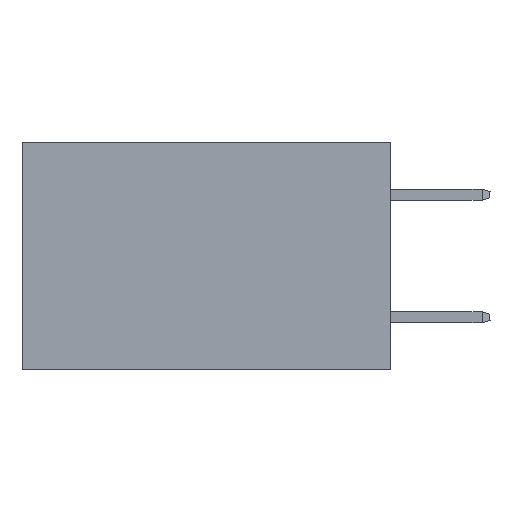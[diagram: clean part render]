
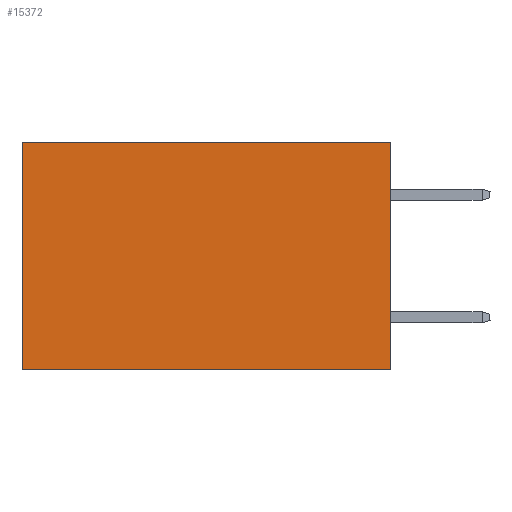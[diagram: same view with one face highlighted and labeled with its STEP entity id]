
A CAD part, left-side view. The second image highlights one B-rep face of the part: STEP entity #15372.
In plain terms, the highlighted planar face has unit normal (-1, 0, 0).
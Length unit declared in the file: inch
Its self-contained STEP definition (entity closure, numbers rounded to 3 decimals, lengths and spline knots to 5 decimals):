
#166 = CARTESIAN_POINT ( 'NONE',  ( 0.2875, 0., 0. ) ) ;
#623 = LINE ( 'NONE', #166, #16661 ) ;
#1208 = DIRECTION ( 'NONE',  ( 0., 0., -1. ) ) ;
#1688 = PLANE ( 'NONE',  #29079 ) ;
#3999 = CARTESIAN_POINT ( 'NONE',  ( 0.2875, 0., 0. ) ) ;
#4594 = EDGE_CURVE ( 'NONE', #4764, #20289, #623, .T. ) ;
#4764 = VERTEX_POINT ( 'NONE', #3999 ) ;
#5933 = ORIENTED_EDGE ( 'NONE', *, *, #18260, .F. ) ;
#6297 = CARTESIAN_POINT ( 'NONE',  ( 0.2875, 0., 0. ) ) ;
#6328 = DIRECTION ( 'NONE',  ( 0., 1., 0. ) ) ;
#7002 = CARTESIAN_POINT ( 'NONE',  ( 0.2875, 0., 0. ) ) ;
#7034 = CARTESIAN_POINT ( 'NONE',  ( 0.2875, 0., -0.37 ) ) ;
#7467 = ORIENTED_EDGE ( 'NONE', *, *, #11620, .T. ) ;
#8313 = EDGE_CURVE ( 'NONE', #12426, #24381, #10343, .T. ) ;
#8551 = ORIENTED_EDGE ( 'NONE', *, *, #4594, .F. ) ;
#10343 = LINE ( 'NONE', #26751, #16919 ) ;
#11377 = LINE ( 'NONE', #17718, #19391 ) ;
#11620 = EDGE_CURVE ( 'NONE', #4764, #12426, #26541, .T. ) ;
#11766 = DIRECTION ( 'NONE',  ( 0., 0., -1. ) ) ;
#12426 = VERTEX_POINT ( 'NONE', #14654 ) ;
#14654 = CARTESIAN_POINT ( 'NONE',  ( 0.2875, 0.6, 0. ) ) ;
#14893 = VECTOR ( 'NONE', #16643, 39.37008 ) ;
#15372 = ADVANCED_FACE ( 'NONE', ( #19197 ), #1688, .F. ) ;
#16643 = DIRECTION ( 'NONE',  ( 0., 1., 0. ) ) ;
#16661 = VECTOR ( 'NONE', #11766, 39.37008 ) ;
#16919 = VECTOR ( 'NONE', #1208, 39.37008 ) ;
#17718 = CARTESIAN_POINT ( 'NONE',  ( 0.2875, 0., -0.37 ) ) ;
#18260 = EDGE_CURVE ( 'NONE', #20289, #24381, #11377, .T. ) ;
#19197 = FACE_OUTER_BOUND ( 'NONE', #24681, .T. ) ;
#19391 = VECTOR ( 'NONE', #6328, 39.37008 ) ;
#19816 = DIRECTION ( 'NONE',  ( 1., 0., 0. ) ) ;
#20289 = VERTEX_POINT ( 'NONE', #7034 ) ;
#22133 = DIRECTION ( 'NONE',  ( 0., 0., -1. ) ) ;
#22860 = ORIENTED_EDGE ( 'NONE', *, *, #8313, .T. ) ;
#24381 = VERTEX_POINT ( 'NONE', #26674 ) ;
#24681 = EDGE_LOOP ( 'NONE', ( #22860, #5933, #8551, #7467 ) ) ;
#26541 = LINE ( 'NONE', #7002, #14893 ) ;
#26674 = CARTESIAN_POINT ( 'NONE',  ( 0.2875, 0.6, -0.37 ) ) ;
#26751 = CARTESIAN_POINT ( 'NONE',  ( 0.2875, 0.6, 0. ) ) ;
#29079 = AXIS2_PLACEMENT_3D ( 'NONE', #6297, #19816, #22133 ) ;
